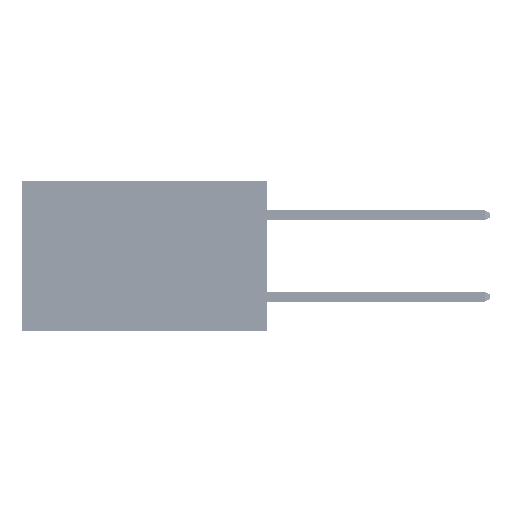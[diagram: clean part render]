
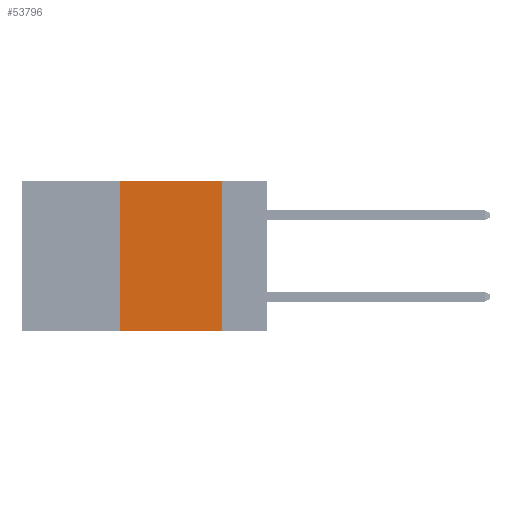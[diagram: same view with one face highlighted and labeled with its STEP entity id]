
A CAD part, left-side view. The second image highlights one B-rep face of the part: STEP entity #53796.
In plain terms, the highlighted planar face has unit normal (-1, 0, 0).
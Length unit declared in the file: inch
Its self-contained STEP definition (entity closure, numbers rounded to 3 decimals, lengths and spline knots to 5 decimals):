
#2317 = CARTESIAN_POINT ( 'NONE',  ( 0., 0.6, 0. ) ) ;
#2690 = CARTESIAN_POINT ( 'NONE',  ( 0., 0.36, 0. ) ) ;
#6460 = DIRECTION ( 'NONE',  ( 0., 0., -1. ) ) ;
#8226 = DIRECTION ( 'NONE',  ( 0., 0., -1. ) ) ;
#8876 = VECTOR ( 'NONE', #44629, 39.37008 ) ;
#11182 = CARTESIAN_POINT ( 'NONE',  ( 0., 0.6, -0.37 ) ) ;
#12190 = CARTESIAN_POINT ( 'NONE',  ( 0., 0.11, 0. ) ) ;
#14668 = ORIENTED_EDGE ( 'NONE', *, *, #25197, .F. ) ;
#15138 = DIRECTION ( 'NONE',  ( 0., -1., 0. ) ) ;
#15993 = ORIENTED_EDGE ( 'NONE', *, *, #42562, .T. ) ;
#16308 = VERTEX_POINT ( 'NONE', #41885 ) ;
#17314 = CARTESIAN_POINT ( 'NONE',  ( 0., 0.11, -0.37 ) ) ;
#19283 = VERTEX_POINT ( 'NONE', #41938 ) ;
#19560 = CARTESIAN_POINT ( 'NONE',  ( 0., 0.6, 0. ) ) ;
#21910 = ORIENTED_EDGE ( 'NONE', *, *, #45084, .F. ) ;
#25197 = EDGE_CURVE ( 'NONE', #32677, #19283, #39722, .T. ) ;
#26826 = CARTESIAN_POINT ( 'NONE',  ( 0., 0.36, 0. ) ) ;
#27310 = PLANE ( 'NONE',  #43865 ) ;
#27854 = VERTEX_POINT ( 'NONE', #17314 ) ;
#29013 = EDGE_CURVE ( 'NONE', #16308, #32677, #43652, .T. ) ;
#31493 = DIRECTION ( 'NONE',  ( 1., 0., 0. ) ) ;
#32598 = VECTOR ( 'NONE', #35225, 39.37008 ) ;
#32677 = VERTEX_POINT ( 'NONE', #2690 ) ;
#35225 = DIRECTION ( 'NONE',  ( 0., 0., 1. ) ) ;
#39565 = VECTOR ( 'NONE', #8226, 39.37008 ) ;
#39722 = LINE ( 'NONE', #19560, #51994 ) ;
#41885 = CARTESIAN_POINT ( 'NONE',  ( 0., 0.36, -0.37 ) ) ;
#41938 = CARTESIAN_POINT ( 'NONE',  ( 0., 0.11, 0. ) ) ;
#42226 = LINE ( 'NONE', #11182, #8876 ) ;
#42562 = EDGE_CURVE ( 'NONE', #16308, #27854, #42226, .T. ) ;
#43652 = LINE ( 'NONE', #26826, #32598 ) ;
#43865 = AXIS2_PLACEMENT_3D ( 'NONE', #2317, #31493, #6460 ) ;
#44629 = DIRECTION ( 'NONE',  ( 0., -1., 0. ) ) ;
#45084 = EDGE_CURVE ( 'NONE', #19283, #27854, #50554, .T. ) ;
#46865 = EDGE_LOOP ( 'NONE', ( #21910, #14668, #47995, #15993 ) ) ;
#47995 = ORIENTED_EDGE ( 'NONE', *, *, #29013, .F. ) ;
#50554 = LINE ( 'NONE', #12190, #39565 ) ;
#51994 = VECTOR ( 'NONE', #15138, 39.37008 ) ;
#52338 = FACE_OUTER_BOUND ( 'NONE', #46865, .T. ) ;
#53796 = ADVANCED_FACE ( 'NONE', ( #52338 ), #27310, .F. ) ;
